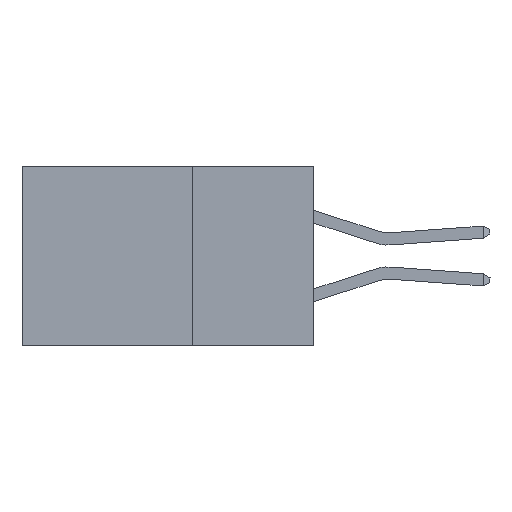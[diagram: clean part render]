
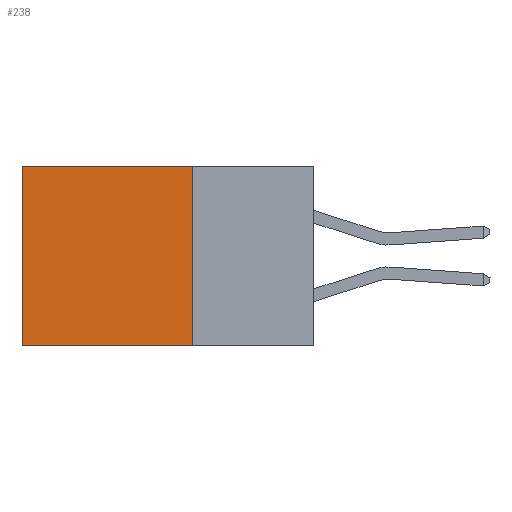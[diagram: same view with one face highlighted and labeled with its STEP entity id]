
A CAD part, left-side view. The second image highlights one B-rep face of the part: STEP entity #238.
In plain terms, the highlighted planar face has unit normal (-1, 0, 0).
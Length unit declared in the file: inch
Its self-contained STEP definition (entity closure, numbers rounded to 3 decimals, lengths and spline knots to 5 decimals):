
#160 = AXIS2_PLACEMENT_3D ( 'NONE', #5494, #13872, #17757 ) ;
#238 = ADVANCED_FACE ( 'NONE', ( #7361 ), #4771, .F. ) ;
#605 = ORIENTED_EDGE ( 'NONE', *, *, #13216, .F. ) ;
#798 = CARTESIAN_POINT ( 'NONE',  ( 0.2875, 0.25, 0. ) ) ;
#1437 = VECTOR ( 'NONE', #9047, 39.37008 ) ;
#1747 = CARTESIAN_POINT ( 'NONE',  ( 0.2875, 0.6, -0.37 ) ) ;
#3253 = EDGE_CURVE ( 'NONE', #4477, #6431, #8317, .T. ) ;
#3890 = CARTESIAN_POINT ( 'NONE',  ( 0.2875, 0.6, 0. ) ) ;
#3979 = ORIENTED_EDGE ( 'NONE', *, *, #3253, .F. ) ;
#4208 = CARTESIAN_POINT ( 'NONE',  ( 0.2875, 0.25, -0.37 ) ) ;
#4477 = VERTEX_POINT ( 'NONE', #17918 ) ;
#4771 = PLANE ( 'NONE',  #160 ) ;
#5074 = DIRECTION ( 'NONE',  ( 0., 0., -1. ) ) ;
#5494 = CARTESIAN_POINT ( 'NONE',  ( 0.2875, 0.25, 0. ) ) ;
#5809 = VECTOR ( 'NONE', #6459, 39.37008 ) ;
#5856 = DIRECTION ( 'NONE',  ( 0., 1., 0. ) ) ;
#5883 = LINE ( 'NONE', #18839, #1437 ) ;
#6373 = LINE ( 'NONE', #798, #9262 ) ;
#6431 = VERTEX_POINT ( 'NONE', #4208 ) ;
#6459 = DIRECTION ( 'NONE',  ( 0., 0., -1. ) ) ;
#6880 = ORIENTED_EDGE ( 'NONE', *, *, #14164, .T. ) ;
#7361 = FACE_OUTER_BOUND ( 'NONE', #13468, .T. ) ;
#7404 = EDGE_CURVE ( 'NONE', #15877, #17242, #18943, .T. ) ;
#7848 = ORIENTED_EDGE ( 'NONE', *, *, #7404, .T. ) ;
#8317 = LINE ( 'NONE', #14993, #17066 ) ;
#9047 = DIRECTION ( 'NONE',  ( 0., 1., 0. ) ) ;
#9262 = VECTOR ( 'NONE', #5856, 39.37008 ) ;
#13216 = EDGE_CURVE ( 'NONE', #6431, #17242, #5883, .T. ) ;
#13468 = EDGE_LOOP ( 'NONE', ( #7848, #605, #3979, #6880 ) ) ;
#13872 = DIRECTION ( 'NONE',  ( 1., 0., 0. ) ) ;
#14164 = EDGE_CURVE ( 'NONE', #4477, #15877, #6373, .T. ) ;
#14993 = CARTESIAN_POINT ( 'NONE',  ( 0.2875, 0.25, 0. ) ) ;
#15877 = VERTEX_POINT ( 'NONE', #3890 ) ;
#17066 = VECTOR ( 'NONE', #5074, 39.37008 ) ;
#17242 = VERTEX_POINT ( 'NONE', #1747 ) ;
#17757 = DIRECTION ( 'NONE',  ( 0., 0., -1. ) ) ;
#17918 = CARTESIAN_POINT ( 'NONE',  ( 0.2875, 0.25, 0. ) ) ;
#18839 = CARTESIAN_POINT ( 'NONE',  ( 0.2875, 0.25, -0.37 ) ) ;
#18943 = LINE ( 'NONE', #21189, #5809 ) ;
#21189 = CARTESIAN_POINT ( 'NONE',  ( 0.2875, 0.6, 0. ) ) ;
